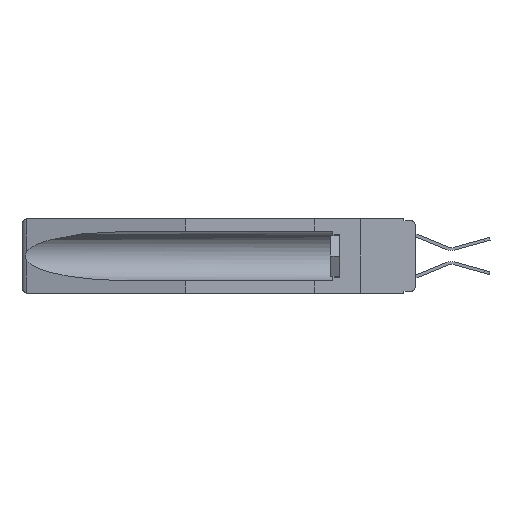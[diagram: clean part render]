
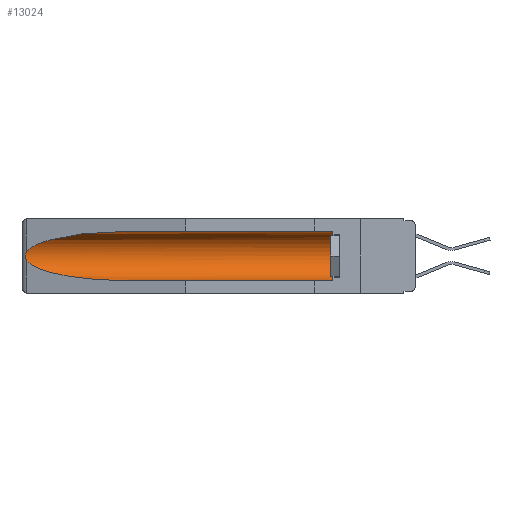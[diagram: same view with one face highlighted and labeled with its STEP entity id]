
A CAD part, left-side view. The second image highlights one B-rep face of the part: STEP entity #13024.
In plain terms, the highlighted cylindrical face has radius 2.857 mm (diameter 5.715 mm), a partial arc.
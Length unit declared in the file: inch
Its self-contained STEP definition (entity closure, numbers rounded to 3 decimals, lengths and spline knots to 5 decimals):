
#985 = CARTESIAN_POINT ( 'NONE',  ( 0.25451, 1.48313, -0.24835 ) ) ;
#2651 = DIRECTION ( 'NONE',  ( 0., 1., 0. ) ) ;
#2783 = CARTESIAN_POINT ( 'NONE',  ( 0.155, -0.30754, -0.284 ) ) ;
#3598 = CARTESIAN_POINT ( 'NONE',  ( 0.26537, 1.52718, -0.19328 ) ) ;
#3723 = CARTESIAN_POINT ( 'NONE',  ( 0.26655, 1.53094, -0.18657 ) ) ;
#4159 = EDGE_CURVE ( 'NONE', #12559, #19197, #18660, .T. ) ;
#4217 = EDGE_CURVE ( 'NONE', #4830, #12559, #19103, .T. ) ;
#4810 = VERTEX_POINT ( 'NONE', #12851 ) ;
#4830 = VERTEX_POINT ( 'NONE', #8520 ) ;
#6230 =( BOUNDED_CURVE ( )  B_SPLINE_CURVE ( 3, ( #18612, #985, #8870, #16686 ),
 .UNSPECIFIED., .F., .F. ) 
 B_SPLINE_CURVE_WITH_KNOTS ( ( 4, 4 ),
 ( 0.1948, 1.5708 ),
 .UNSPECIFIED. ) 
 CURVE ( )  GEOMETRIC_REPRESENTATION_ITEM ( )  RATIONAL_B_SPLINE_CURVE ( ( 1., 0.848, 0.848, 1. ) ) 
 REPRESENTATION_ITEM ( '' )  );
#6257 = EDGE_CURVE ( 'NONE', #19197, #4810, #13699, .T. ) ;
#6929 = DIRECTION ( 'NONE',  ( 0., 1., 0. ) ) ;
#7627 = CARTESIAN_POINT ( 'NONE',  ( 0.26654, 1.53092, -0.15636 ) ) ;
#7806 = CARTESIAN_POINT ( 'NONE',  ( 0.21114, 1.30732, -0.059 ) ) ;
#8044 = VECTOR ( 'NONE', #9843, 39.37008 ) ;
#8520 = CARTESIAN_POINT ( 'NONE',  ( 0.155, 0.126, -0.059 ) ) ;
#8870 = CARTESIAN_POINT ( 'NONE',  ( 0.21114, 1.30732, -0.284 ) ) ;
#9833 = VERTEX_POINT ( 'NONE', #12642 ) ;
#9843 = DIRECTION ( 'NONE',  ( 0., 1., 0. ) ) ;
#11072 = CARTESIAN_POINT ( 'NONE',  ( 0.26597, 1.52961, -0.15275 ) ) ;
#11414 = FACE_OUTER_BOUND ( 'NONE', #16220, .T. ) ;
#12559 = VERTEX_POINT ( 'NONE', #20746 ) ;
#12633 = ORIENTED_EDGE ( 'NONE', *, *, #14537, .T. ) ;
#12642 = CARTESIAN_POINT ( 'NONE',  ( 0.155, 1.07973, -0.284 ) ) ;
#12851 = CARTESIAN_POINT ( 'NONE',  ( 0.26537, 1.52718, -0.19328 ) ) ;
#13024 = ADVANCED_FACE ( 'NONE', ( #11414 ), #22924, .F. ) ;
#13079 = VECTOR ( 'NONE', #2651, 39.37008 ) ;
#13699 = B_SPLINE_CURVE_WITH_KNOTS ( 'NONE', 3,
 ( #15064, #11072, #7627, #21345, #24779, #17491, #16984, #3723, #21222, #3598 ),
 .UNSPECIFIED., .F., .F.,
 ( 4, 2, 2, 2, 4 ),
 ( 0., 0.00029, 0.00058, 0.00087, 0.00117 ),
 .UNSPECIFIED. ) ;
#14428 = ORIENTED_EDGE ( 'NONE', *, *, #21406, .T. ) ;
#14458 = VERTEX_POINT ( 'NONE', #18738 ) ;
#14537 = EDGE_CURVE ( 'NONE', #14458, #4830, #16241, .T. ) ;
#14691 = AXIS2_PLACEMENT_3D ( 'NONE', #14752, #6929, #24598 ) ;
#14712 = ORIENTED_EDGE ( 'NONE', *, *, #6257, .T. ) ;
#14752 = CARTESIAN_POINT ( 'NONE',  ( 0.155, -0.30754, -0.1715 ) ) ;
#14884 = DIRECTION ( 'NONE',  ( 0., 0., 1. ) ) ;
#15064 = CARTESIAN_POINT ( 'NONE',  ( 0.26537, 1.52718, -0.14972 ) ) ;
#15238 = CARTESIAN_POINT ( 'NONE',  ( 0.25451, 1.48313, -0.09465 ) ) ;
#15687 = ORIENTED_EDGE ( 'NONE', *, *, #4159, .T. ) ;
#16220 = EDGE_LOOP ( 'NONE', ( #15687, #14712, #14428, #24377, #12633, #17921 ) ) ;
#16241 = CIRCLE ( 'NONE', #24813, 0.1125 ) ;
#16686 = CARTESIAN_POINT ( 'NONE',  ( 0.155, 1.07973, -0.284 ) ) ;
#16937 = CARTESIAN_POINT ( 'NONE',  ( 0.155, 0.126, -0.1715 ) ) ;
#16984 = CARTESIAN_POINT ( 'NONE',  ( 0.2673, 1.53269, -0.17917 ) ) ;
#17174 = CARTESIAN_POINT ( 'NONE',  ( 0.26537, 1.52718, -0.14972 ) ) ;
#17479 = EDGE_CURVE ( 'NONE', #14458, #9833, #18496, .T. ) ;
#17491 = CARTESIAN_POINT ( 'NONE',  ( 0.2675, 1.53308, -0.17534 ) ) ;
#17921 = ORIENTED_EDGE ( 'NONE', *, *, #4217, .T. ) ;
#18496 = LINE ( 'NONE', #2783, #13079 ) ;
#18612 = CARTESIAN_POINT ( 'NONE',  ( 0.26537, 1.52718, -0.19328 ) ) ;
#18660 =( BOUNDED_CURVE ( )  B_SPLINE_CURVE ( 3, ( #25102, #7806, #15238, #17174 ),
 .UNSPECIFIED., .F., .F. ) 
 B_SPLINE_CURVE_WITH_KNOTS ( ( 4, 4 ),
 ( 4.71239, 6.08839 ),
 .UNSPECIFIED. ) 
 CURVE ( )  GEOMETRIC_REPRESENTATION_ITEM ( )  RATIONAL_B_SPLINE_CURVE ( ( 1., 0.848, 0.848, 1. ) ) 
 REPRESENTATION_ITEM ( '' )  );
#18738 = CARTESIAN_POINT ( 'NONE',  ( 0.155, 0.126, -0.284 ) ) ;
#19103 = LINE ( 'NONE', #24977, #8044 ) ;
#19197 = VERTEX_POINT ( 'NONE', #23840 ) ;
#19245 = DIRECTION ( 'NONE',  ( 0., -1., 0. ) ) ;
#20746 = CARTESIAN_POINT ( 'NONE',  ( 0.155, 1.07973, -0.059 ) ) ;
#21222 = CARTESIAN_POINT ( 'NONE',  ( 0.26597, 1.5296, -0.19026 ) ) ;
#21345 = CARTESIAN_POINT ( 'NONE',  ( 0.2673, 1.5327, -0.16383 ) ) ;
#21406 = EDGE_CURVE ( 'NONE', #4810, #9833, #6230, .T. ) ;
#22924 = CYLINDRICAL_SURFACE ( 'NONE', #14691, 0.1125 ) ;
#23840 = CARTESIAN_POINT ( 'NONE',  ( 0.26537, 1.52718, -0.14972 ) ) ;
#24377 = ORIENTED_EDGE ( 'NONE', *, *, #17479, .F. ) ;
#24598 = DIRECTION ( 'NONE',  ( 0., 0., 1. ) ) ;
#24779 = CARTESIAN_POINT ( 'NONE',  ( 0.2675, 1.53308, -0.16763 ) ) ;
#24813 = AXIS2_PLACEMENT_3D ( 'NONE', #16937, #19245, #14884 ) ;
#24977 = CARTESIAN_POINT ( 'NONE',  ( 0.155, -0.30754, -0.059 ) ) ;
#25102 = CARTESIAN_POINT ( 'NONE',  ( 0.155, 1.07973, -0.059 ) ) ;
